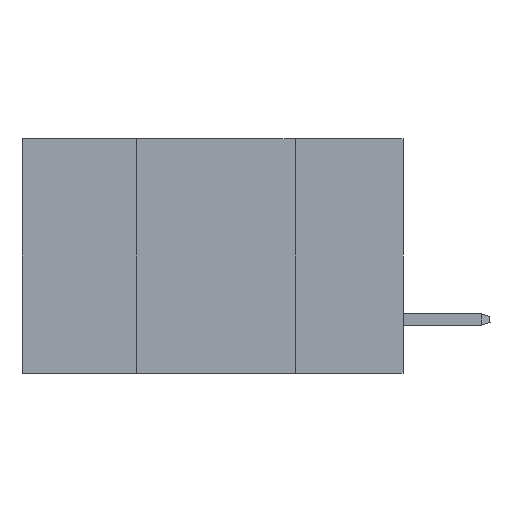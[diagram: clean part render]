
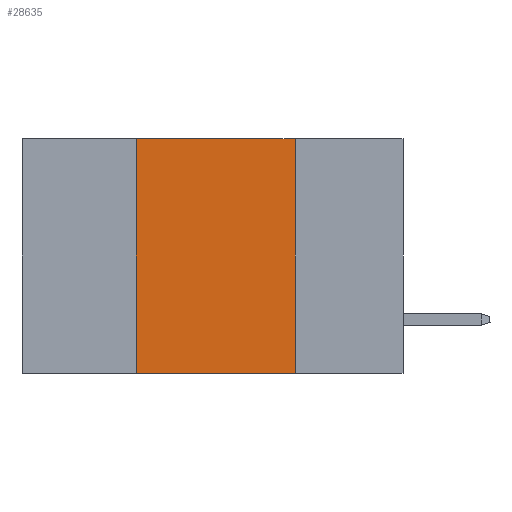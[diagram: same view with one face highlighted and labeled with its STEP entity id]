
A CAD part, left-side view. The second image highlights one B-rep face of the part: STEP entity #28635.
In plain terms, the highlighted planar face has unit normal (-1, 0, 0).
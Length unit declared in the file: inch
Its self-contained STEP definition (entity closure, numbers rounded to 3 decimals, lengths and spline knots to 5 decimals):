
#610 = EDGE_CURVE ( 'NONE', #20120, #25963, #9464, .T. ) ;
#1417 = ORIENTED_EDGE ( 'NONE', *, *, #610, .F. ) ;
#1914 = DIRECTION ( 'NONE',  ( 0., 0., -1. ) ) ;
#1938 = VECTOR ( 'NONE', #3550, 39.37008 ) ;
#2085 = LINE ( 'NONE', #13598, #21463 ) ;
#2907 = AXIS2_PLACEMENT_3D ( 'NONE', #24932, #29529, #15345 ) ;
#3550 = DIRECTION ( 'NONE',  ( 0., -1., 0. ) ) ;
#4193 = VECTOR ( 'NONE', #1914, 39.37008 ) ;
#5312 = LINE ( 'NONE', #27198, #1938 ) ;
#6347 = CARTESIAN_POINT ( 'NONE',  ( 0., 0.42, 0. ) ) ;
#6616 = CARTESIAN_POINT ( 'NONE',  ( 0., 0.42, -0.37 ) ) ;
#7099 = DIRECTION ( 'NONE',  ( 0., -1., 0. ) ) ;
#7523 = EDGE_CURVE ( 'NONE', #27174, #20120, #5312, .T. ) ;
#9464 = LINE ( 'NONE', #23502, #4193 ) ;
#11802 = CARTESIAN_POINT ( 'NONE',  ( 0., 0.17, -0.37 ) ) ;
#13294 = VECTOR ( 'NONE', #15499, 39.37008 ) ;
#13469 = EDGE_LOOP ( 'NONE', ( #1417, #23991, #26790, #19559 ) ) ;
#13598 = CARTESIAN_POINT ( 'NONE',  ( 0., 0.6, -0.37 ) ) ;
#14479 = EDGE_CURVE ( 'NONE', #24708, #25963, #2085, .T. ) ;
#15345 = DIRECTION ( 'NONE',  ( 0., 0., -1. ) ) ;
#15499 = DIRECTION ( 'NONE',  ( 0., 0., 1. ) ) ;
#17414 = FACE_OUTER_BOUND ( 'NONE', #13469, .T. ) ;
#19450 = CARTESIAN_POINT ( 'NONE',  ( 0., 0.42, 0. ) ) ;
#19559 = ORIENTED_EDGE ( 'NONE', *, *, #14479, .T. ) ;
#19917 = PLANE ( 'NONE',  #2907 ) ;
#20120 = VERTEX_POINT ( 'NONE', #26733 ) ;
#21463 = VECTOR ( 'NONE', #7099, 39.37008 ) ;
#22936 = EDGE_CURVE ( 'NONE', #24708, #27174, #29842, .T. ) ;
#23502 = CARTESIAN_POINT ( 'NONE',  ( 0., 0.17, 0. ) ) ;
#23991 = ORIENTED_EDGE ( 'NONE', *, *, #7523, .F. ) ;
#24708 = VERTEX_POINT ( 'NONE', #6616 ) ;
#24932 = CARTESIAN_POINT ( 'NONE',  ( 0., 0.6, 0. ) ) ;
#25963 = VERTEX_POINT ( 'NONE', #11802 ) ;
#26733 = CARTESIAN_POINT ( 'NONE',  ( 0., 0.17, 0. ) ) ;
#26790 = ORIENTED_EDGE ( 'NONE', *, *, #22936, .F. ) ;
#27174 = VERTEX_POINT ( 'NONE', #19450 ) ;
#27198 = CARTESIAN_POINT ( 'NONE',  ( 0., 0.6, 0. ) ) ;
#28635 = ADVANCED_FACE ( 'NONE', ( #17414 ), #19917, .F. ) ;
#29529 = DIRECTION ( 'NONE',  ( 1., 0., 0. ) ) ;
#29842 = LINE ( 'NONE', #6347, #13294 ) ;
